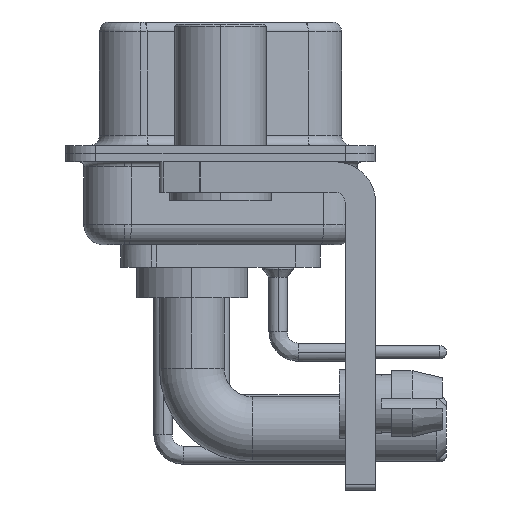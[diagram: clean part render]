
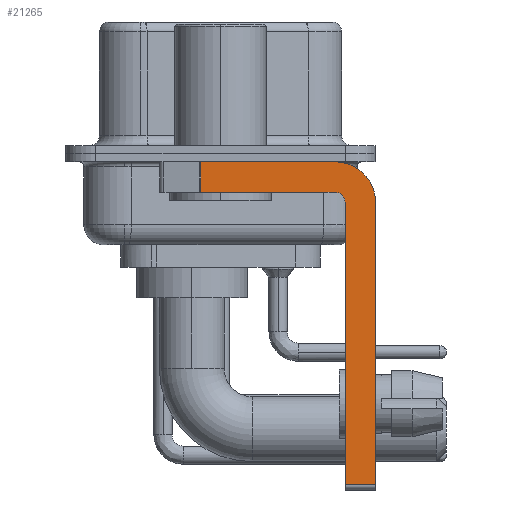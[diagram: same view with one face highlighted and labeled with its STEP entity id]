
A CAD part, left-side view. The second image highlights one B-rep face of the part: STEP entity #21265.
In plain terms, the highlighted planar face has unit normal (-1, 0, 0).
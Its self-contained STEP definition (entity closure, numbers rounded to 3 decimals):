
#425 = DIRECTION ( 'NONE',  ( 0., 0., -1. ) ) ;
#503 = VECTOR ( 'NONE', #36655, 1000. ) ;
#855 = AXIS2_PLACEMENT_3D ( 'NONE', #23375, #31335, #4734 ) ;
#1926 = DIRECTION ( 'NONE',  ( 1., 0., 0. ) ) ;
#2401 = VECTOR ( 'NONE', #425, 1000. ) ;
#2556 = LINE ( 'NONE', #34802, #35039 ) ;
#2688 = DIRECTION ( 'NONE',  ( 0., 1., 0. ) ) ;
#3815 = DIRECTION ( 'NONE',  ( 0., -1., 0. ) ) ;
#4734 = DIRECTION ( 'NONE',  ( 0., 0., 1. ) ) ;
#4846 = CARTESIAN_POINT ( 'NONE',  ( -2.9, -5.65, -2.4 ) ) ;
#6262 = ORIENTED_EDGE ( 'NONE', *, *, #22573, .T. ) ;
#6607 = DIRECTION ( 'NONE',  ( 1., 0., 0. ) ) ;
#6687 = AXIS2_PLACEMENT_3D ( 'NONE', #33205, #6607, #8965 ) ;
#8095 = EDGE_LOOP ( 'NONE', ( #15337, #9570, #13132, #8285, #27811, #6262, #31090, #28394 ) ) ;
#8285 = ORIENTED_EDGE ( 'NONE', *, *, #19145, .F. ) ;
#8817 = VERTEX_POINT ( 'NONE', #29781 ) ;
#8965 = DIRECTION ( 'NONE',  ( 0., 0., -1. ) ) ;
#9162 = EDGE_CURVE ( 'NONE', #37517, #32460, #13939, .T. ) ;
#9570 = ORIENTED_EDGE ( 'NONE', *, *, #12133, .T. ) ;
#9647 = LINE ( 'NONE', #21503, #14630 ) ;
#10385 = CARTESIAN_POINT ( 'NONE',  ( -2.9, -6.15, -16.35 ) ) ;
#10640 = CARTESIAN_POINT ( 'NONE',  ( -2.9, 0.978, -1.9 ) ) ;
#11373 = CARTESIAN_POINT ( 'NONE',  ( -2.9, -7.65, -2.4 ) ) ;
#12133 = EDGE_CURVE ( 'NONE', #37517, #24427, #22293, .T. ) ;
#12502 = VERTEX_POINT ( 'NONE', #16017 ) ;
#12853 = CIRCLE ( 'NONE', #6687, 2. ) ;
#13132 = ORIENTED_EDGE ( 'NONE', *, *, #18137, .F. ) ;
#13939 = LINE ( 'NONE', #28717, #37259 ) ;
#14585 = DIRECTION ( 'NONE',  ( 0., 0., 1. ) ) ;
#14630 = VECTOR ( 'NONE', #3815, 1000. ) ;
#15053 = VERTEX_POINT ( 'NONE', #10385 ) ;
#15337 = ORIENTED_EDGE ( 'NONE', *, *, #9162, .F. ) ;
#15855 = AXIS2_PLACEMENT_3D ( 'NONE', #4846, #1926, #34552 ) ;
#16017 = CARTESIAN_POINT ( 'NONE',  ( -2.9, -6.15, -2.4 ) ) ;
#18137 = EDGE_CURVE ( 'NONE', #29126, #24427, #32015, .T. ) ;
#18413 = CARTESIAN_POINT ( 'NONE',  ( -2.9, -5.65, -0.4 ) ) ;
#19145 = EDGE_CURVE ( 'NONE', #12502, #29126, #23797, .T. ) ;
#19583 = DIRECTION ( 'NONE',  ( 0., -1., 0. ) ) ;
#19600 = FACE_OUTER_BOUND ( 'NONE', #8095, .T. ) ;
#21265 = ADVANCED_FACE ( 'NONE', ( #19600 ), #34752, .F. ) ;
#21503 = CARTESIAN_POINT ( 'NONE',  ( -2.9, -5.65, -16.35 ) ) ;
#21930 = EDGE_CURVE ( 'NONE', #15053, #12502, #2556, .T. ) ;
#22293 = LINE ( 'NONE', #10640, #503 ) ;
#22573 = EDGE_CURVE ( 'NONE', #15053, #8817, #9647, .T. ) ;
#23375 = CARTESIAN_POINT ( 'NONE',  ( -2.9, -5.65, -2.4 ) ) ;
#23797 = CIRCLE ( 'NONE', #855, 0.5 ) ;
#24427 = VERTEX_POINT ( 'NONE', #34428 ) ;
#26724 = EDGE_CURVE ( 'NONE', #34662, #8817, #33241, .T. ) ;
#27811 = ORIENTED_EDGE ( 'NONE', *, *, #21930, .F. ) ;
#28074 = VECTOR ( 'NONE', #2688, 1000. ) ;
#28394 = ORIENTED_EDGE ( 'NONE', *, *, #35282, .F. ) ;
#28717 = CARTESIAN_POINT ( 'NONE',  ( -2.9, 3., -0.4 ) ) ;
#29126 = VERTEX_POINT ( 'NONE', #37478 ) ;
#29781 = CARTESIAN_POINT ( 'NONE',  ( -2.9, -7.65, -16.35 ) ) ;
#31090 = ORIENTED_EDGE ( 'NONE', *, *, #26724, .F. ) ;
#31335 = DIRECTION ( 'NONE',  ( -1., 0., 0. ) ) ;
#32015 = LINE ( 'NONE', #37821, #28074 ) ;
#32460 = VERTEX_POINT ( 'NONE', #18413 ) ;
#33205 = CARTESIAN_POINT ( 'NONE',  ( -2.9, -5.65, -2.4 ) ) ;
#33241 = LINE ( 'NONE', #11373, #2401 ) ;
#34428 = CARTESIAN_POINT ( 'NONE',  ( -2.9, 0.978, -1.9 ) ) ;
#34552 = DIRECTION ( 'NONE',  ( 0., 0., -1. ) ) ;
#34662 = VERTEX_POINT ( 'NONE', #37558 ) ;
#34752 = PLANE ( 'NONE',  #15855 ) ;
#34802 = CARTESIAN_POINT ( 'NONE',  ( -2.9, -6.15, -16.6 ) ) ;
#35039 = VECTOR ( 'NONE', #14585, 1000. ) ;
#35282 = EDGE_CURVE ( 'NONE', #32460, #34662, #12853, .T. ) ;
#36655 = DIRECTION ( 'NONE',  ( 0., 0., -1. ) ) ;
#37250 = CARTESIAN_POINT ( 'NONE',  ( -2.9, 0.978, -0.4 ) ) ;
#37259 = VECTOR ( 'NONE', #19583, 1000. ) ;
#37478 = CARTESIAN_POINT ( 'NONE',  ( -2.9, -5.65, -1.9 ) ) ;
#37517 = VERTEX_POINT ( 'NONE', #37250 ) ;
#37558 = CARTESIAN_POINT ( 'NONE',  ( -2.9, -7.65, -2.4 ) ) ;
#37821 = CARTESIAN_POINT ( 'NONE',  ( -2.9, -5.65, -1.9 ) ) ;
